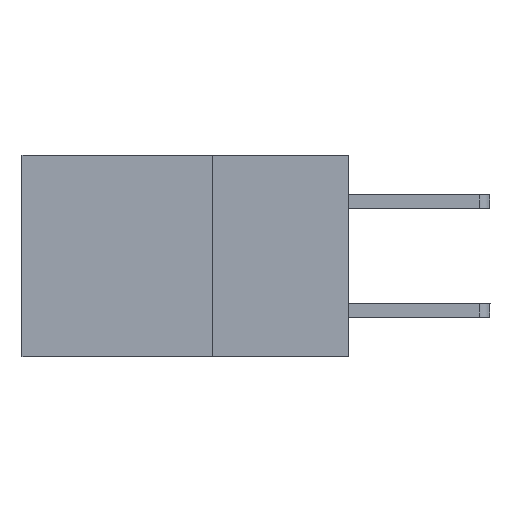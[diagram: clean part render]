
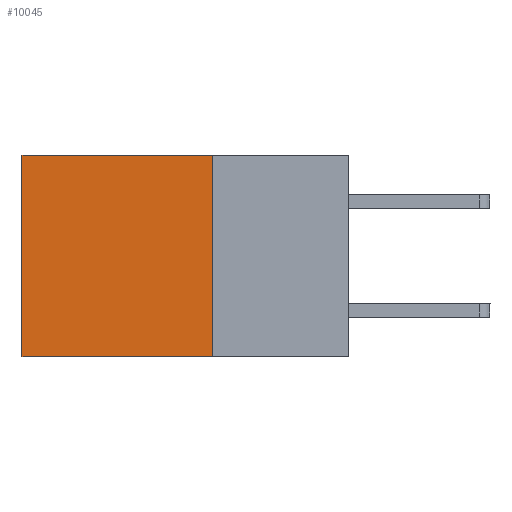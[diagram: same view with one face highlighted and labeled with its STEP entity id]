
A CAD part, left-side view. The second image highlights one B-rep face of the part: STEP entity #10045.
In plain terms, the highlighted planar face has unit normal (-1, 0, 0).
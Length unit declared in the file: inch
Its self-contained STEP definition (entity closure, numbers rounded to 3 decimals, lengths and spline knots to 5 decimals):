
#43 = VERTEX_POINT ( 'NONE', #4198 ) ;
#426 = DIRECTION ( 'NONE',  ( 0., 0., -1. ) ) ;
#454 = CARTESIAN_POINT ( 'NONE',  ( 0.2615, 0.6, -0.37 ) ) ;
#961 = VECTOR ( 'NONE', #2112, 39.37008 ) ;
#1135 = FACE_OUTER_BOUND ( 'NONE', #4419, .T. ) ;
#1248 = VECTOR ( 'NONE', #8821, 39.37008 ) ;
#1560 = CARTESIAN_POINT ( 'NONE',  ( 0.2615, 0.25, -0.37 ) ) ;
#1626 = VERTEX_POINT ( 'NONE', #1560 ) ;
#2075 = LINE ( 'NONE', #7781, #6157 ) ;
#2112 = DIRECTION ( 'NONE',  ( 0., 0., -1. ) ) ;
#2470 = EDGE_CURVE ( 'NONE', #43, #5431, #2075, .T. ) ;
#2481 = ORIENTED_EDGE ( 'NONE', *, *, #3562, .F. ) ;
#3562 = EDGE_CURVE ( 'NONE', #1626, #5252, #5680, .T. ) ;
#4198 = CARTESIAN_POINT ( 'NONE',  ( 0.2615, 0.25, 0. ) ) ;
#4235 = CARTESIAN_POINT ( 'NONE',  ( 0.2615, 0.6, 0. ) ) ;
#4419 = EDGE_LOOP ( 'NONE', ( #8668, #2481, #8192, #5913 ) ) ;
#4620 = EDGE_CURVE ( 'NONE', #5431, #5252, #8478, .T. ) ;
#5078 = PLANE ( 'NONE',  #9340 ) ;
#5214 = EDGE_CURVE ( 'NONE', #43, #1626, #9537, .T. ) ;
#5252 = VERTEX_POINT ( 'NONE', #7745 ) ;
#5431 = VERTEX_POINT ( 'NONE', #4235 ) ;
#5680 = LINE ( 'NONE', #8846, #1248 ) ;
#5861 = DIRECTION ( 'NONE',  ( 0., 0., -1. ) ) ;
#5913 = ORIENTED_EDGE ( 'NONE', *, *, #2470, .T. ) ;
#6157 = VECTOR ( 'NONE', #7683, 39.37008 ) ;
#7683 = DIRECTION ( 'NONE',  ( 0., 1., 0. ) ) ;
#7745 = CARTESIAN_POINT ( 'NONE',  ( 0.2615, 0.6, -0.37 ) ) ;
#7781 = CARTESIAN_POINT ( 'NONE',  ( 0.2615, 0.25, 0. ) ) ;
#8192 = ORIENTED_EDGE ( 'NONE', *, *, #5214, .F. ) ;
#8235 = VECTOR ( 'NONE', #426, 39.37008 ) ;
#8478 = LINE ( 'NONE', #454, #8235 ) ;
#8668 = ORIENTED_EDGE ( 'NONE', *, *, #4620, .T. ) ;
#8779 = CARTESIAN_POINT ( 'NONE',  ( 0.2615, 0.25, -0.37 ) ) ;
#8821 = DIRECTION ( 'NONE',  ( 0., 1., 0. ) ) ;
#8846 = CARTESIAN_POINT ( 'NONE',  ( 0.2615, 0.25, -0.37 ) ) ;
#9340 = AXIS2_PLACEMENT_3D ( 'NONE', #8779, #10162, #5861 ) ;
#9537 = LINE ( 'NONE', #9779, #961 ) ;
#9779 = CARTESIAN_POINT ( 'NONE',  ( 0.2615, 0.25, -0.37 ) ) ;
#10045 = ADVANCED_FACE ( 'NONE', ( #1135 ), #5078, .F. ) ;
#10162 = DIRECTION ( 'NONE',  ( 1., 0., 0. ) ) ;
